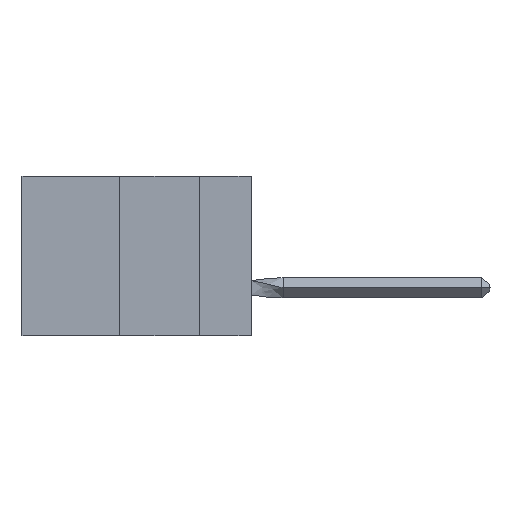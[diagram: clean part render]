
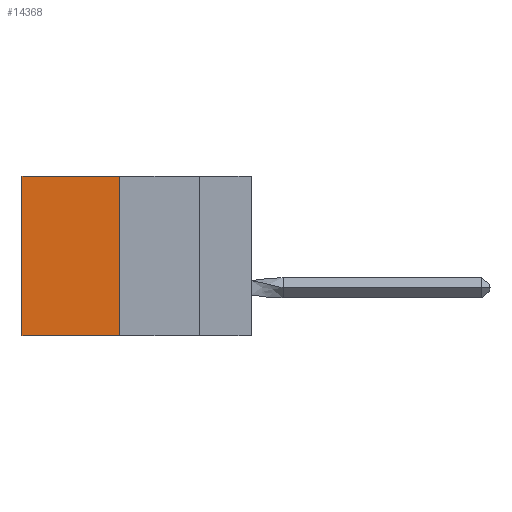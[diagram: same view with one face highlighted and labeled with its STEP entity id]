
A CAD part, left-side view. The second image highlights one B-rep face of the part: STEP entity #14368.
In plain terms, the highlighted planar face has unit normal (-1, 0, 0).
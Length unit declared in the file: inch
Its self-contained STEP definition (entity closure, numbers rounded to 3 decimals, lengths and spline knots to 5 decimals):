
#200 = PLANE ( 'NONE',  #11193 ) ;
#252 = VERTEX_POINT ( 'NONE', #10597 ) ;
#272 = EDGE_CURVE ( 'NONE', #10051, #14549, #16316, .T. ) ;
#1248 = CARTESIAN_POINT ( 'NONE',  ( 0.305, 0.413, -0.5 ) ) ;
#1425 = ORIENTED_EDGE ( 'NONE', *, *, #1428, .F. ) ;
#1428 = EDGE_CURVE ( 'NONE', #11573, #10051, #2077, .T. ) ;
#2077 = LINE ( 'NONE', #1248, #16075 ) ;
#2123 = VECTOR ( 'NONE', #13305, 39.37008 ) ;
#2216 = LINE ( 'NONE', #4847, #4104 ) ;
#2491 = CARTESIAN_POINT ( 'NONE',  ( 0.305, 0.413, -0.5 ) ) ;
#3800 = DIRECTION ( 'NONE',  ( 0., 1., 0. ) ) ;
#3980 = DIRECTION ( 'NONE',  ( 0., 0., -1. ) ) ;
#4104 = VECTOR ( 'NONE', #3800, 39.37008 ) ;
#4513 = DIRECTION ( 'NONE',  ( 0., 0., -1. ) ) ;
#4847 = CARTESIAN_POINT ( 'NONE',  ( 0.305, 0.413, 0. ) ) ;
#5337 = CARTESIAN_POINT ( 'NONE',  ( 0.305, 0.413, -0.5 ) ) ;
#5907 = VECTOR ( 'NONE', #4513, 39.37008 ) ;
#6167 = ORIENTED_EDGE ( 'NONE', *, *, #12301, .T. ) ;
#9515 = LINE ( 'NONE', #14094, #5907 ) ;
#10051 = VERTEX_POINT ( 'NONE', #15456 ) ;
#10597 = CARTESIAN_POINT ( 'NONE',  ( 0.305, 0.72, 0. ) ) ;
#10851 = DIRECTION ( 'NONE',  ( 0., 0., -1. ) ) ;
#11193 = AXIS2_PLACEMENT_3D ( 'NONE', #5337, #12156, #10851 ) ;
#11573 = VERTEX_POINT ( 'NONE', #14846 ) ;
#12156 = DIRECTION ( 'NONE',  ( 1., 0., 0. ) ) ;
#12301 = EDGE_CURVE ( 'NONE', #252, #14549, #9515, .T. ) ;
#13305 = DIRECTION ( 'NONE',  ( 0., 1., 0. ) ) ;
#13712 = FACE_OUTER_BOUND ( 'NONE', #16450, .T. ) ;
#14094 = CARTESIAN_POINT ( 'NONE',  ( 0.305, 0.72, -0.5 ) ) ;
#14368 = ADVANCED_FACE ( 'NONE', ( #13712 ), #200, .F. ) ;
#14549 = VERTEX_POINT ( 'NONE', #15651 ) ;
#14846 = CARTESIAN_POINT ( 'NONE',  ( 0.305, 0.413, 0. ) ) ;
#15456 = CARTESIAN_POINT ( 'NONE',  ( 0.305, 0.413, -0.5 ) ) ;
#15651 = CARTESIAN_POINT ( 'NONE',  ( 0.305, 0.72, -0.5 ) ) ;
#15799 = ORIENTED_EDGE ( 'NONE', *, *, #16465, .T. ) ;
#16075 = VECTOR ( 'NONE', #3980, 39.37008 ) ;
#16287 = ORIENTED_EDGE ( 'NONE', *, *, #272, .F. ) ;
#16316 = LINE ( 'NONE', #2491, #2123 ) ;
#16450 = EDGE_LOOP ( 'NONE', ( #6167, #16287, #1425, #15799 ) ) ;
#16465 = EDGE_CURVE ( 'NONE', #11573, #252, #2216, .T. ) ;
